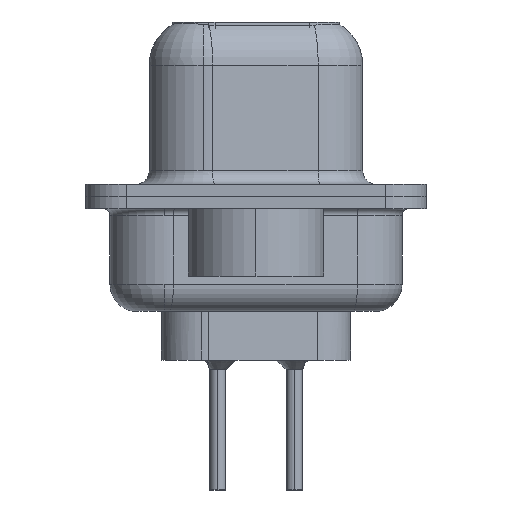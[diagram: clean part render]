
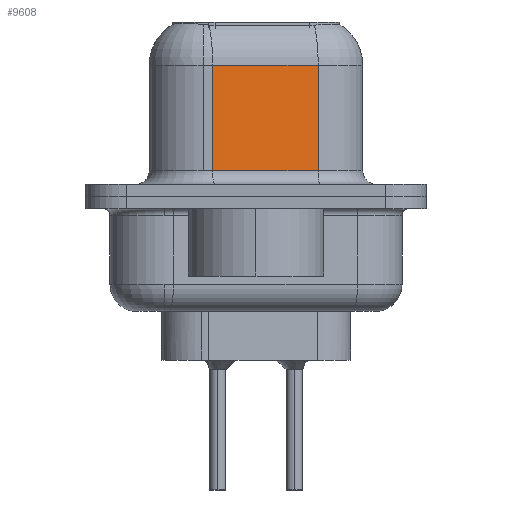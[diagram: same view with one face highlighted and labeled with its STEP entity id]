
A CAD part, left-side view. The second image highlights one B-rep face of the part: STEP entity #9608.
In plain terms, the highlighted planar face has unit normal (-0.985, -0.174, 0).
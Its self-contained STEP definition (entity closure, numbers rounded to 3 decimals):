
#807 = LINE ( 'NONE', #12307, #22952 ) ;
#812 = DIRECTION ( 'NONE',  ( 0., 0., -1. ) ) ;
#1080 = ORIENTED_EDGE ( 'NONE', *, *, #6223, .F. ) ;
#2412 = VERTEX_POINT ( 'NONE', #13496 ) ;
#2652 = CARTESIAN_POINT ( 'NONE',  ( 5.053, -2.297, 6.6 ) ) ;
#4122 = LINE ( 'NONE', #2652, #22797 ) ;
#4349 = VECTOR ( 'NONE', #4630, 1000. ) ;
#4616 = AXIS2_PLACEMENT_3D ( 'NONE', #10382, #17410, #12205 ) ;
#4630 = DIRECTION ( 'NONE',  ( 0.174, -0.985, 0. ) ) ;
#4734 = PLANE ( 'NONE',  #4616 ) ;
#6223 = EDGE_CURVE ( 'NONE', #2412, #12026, #4122, .T. ) ;
#6328 = LINE ( 'NONE', #21309, #4349 ) ;
#7235 = ORIENTED_EDGE ( 'NONE', *, *, #20108, .T. ) ;
#8515 = LINE ( 'NONE', #19440, #9183 ) ;
#9183 = VECTOR ( 'NONE', #21401, 1000. ) ;
#9608 = ADVANCED_FACE ( 'NONE', ( #12089 ), #4734, .F. ) ;
#10382 = CARTESIAN_POINT ( 'NONE',  ( 5.053, -2.297, 6.6 ) ) ;
#12026 = VERTEX_POINT ( 'NONE', #22130 ) ;
#12089 = FACE_OUTER_BOUND ( 'NONE', #20687, .T. ) ;
#12205 = DIRECTION ( 'NONE',  ( -0.174, 0.985, 0. ) ) ;
#12257 = EDGE_CURVE ( 'NONE', #2412, #12841, #807, .T. ) ;
#12307 = CARTESIAN_POINT ( 'NONE',  ( 5.053, -2.297, 4.85 ) ) ;
#12730 = VERTEX_POINT ( 'NONE', #19524 ) ;
#12841 = VERTEX_POINT ( 'NONE', #15665 ) ;
#13496 = CARTESIAN_POINT ( 'NONE',  ( 5.053, -2.297, 4.85 ) ) ;
#14539 = EDGE_CURVE ( 'NONE', #12730, #12026, #6328, .T. ) ;
#15665 = CARTESIAN_POINT ( 'NONE',  ( 4.365, 1.603, 4.85 ) ) ;
#17410 = DIRECTION ( 'NONE',  ( 0.985, 0.174, 0. ) ) ;
#18683 = ORIENTED_EDGE ( 'NONE', *, *, #14539, .T. ) ;
#19440 = CARTESIAN_POINT ( 'NONE',  ( 4.365, 1.603, 6.6 ) ) ;
#19524 = CARTESIAN_POINT ( 'NONE',  ( 4.365, 1.603, 0.95 ) ) ;
#19555 = DIRECTION ( 'NONE',  ( -0.174, 0.985, 0. ) ) ;
#19789 = ORIENTED_EDGE ( 'NONE', *, *, #12257, .T. ) ;
#20108 = EDGE_CURVE ( 'NONE', #12841, #12730, #8515, .T. ) ;
#20687 = EDGE_LOOP ( 'NONE', ( #1080, #19789, #7235, #18683 ) ) ;
#21309 = CARTESIAN_POINT ( 'NONE',  ( 5.053, -2.297, 0.95 ) ) ;
#21401 = DIRECTION ( 'NONE',  ( 0., 0., -1. ) ) ;
#22130 = CARTESIAN_POINT ( 'NONE',  ( 5.053, -2.297, 0.95 ) ) ;
#22797 = VECTOR ( 'NONE', #812, 1000. ) ;
#22952 = VECTOR ( 'NONE', #19555, 1000. ) ;
